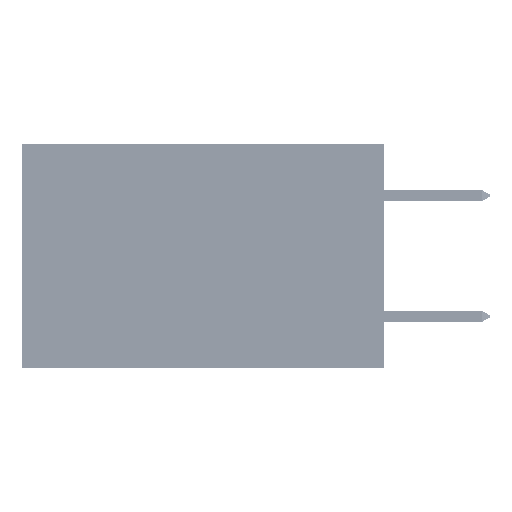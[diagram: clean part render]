
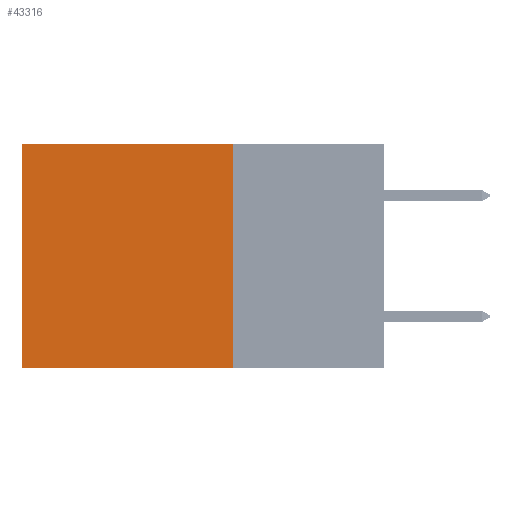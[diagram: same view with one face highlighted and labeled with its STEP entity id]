
A CAD part, left-side view. The second image highlights one B-rep face of the part: STEP entity #43316.
In plain terms, the highlighted planar face has unit normal (-1, 0, 0).
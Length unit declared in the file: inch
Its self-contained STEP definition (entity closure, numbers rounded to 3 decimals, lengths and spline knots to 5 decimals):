
#199 = VERTEX_POINT ( 'NONE', #32326 ) ;
#1847 = PLANE ( 'NONE',  #6595 ) ;
#2545 = VERTEX_POINT ( 'NONE', #3781 ) ;
#2613 = LINE ( 'NONE', #25342, #10153 ) ;
#3607 = ORIENTED_EDGE ( 'NONE', *, *, #38591, .T. ) ;
#3781 = CARTESIAN_POINT ( 'NONE',  ( 0.2875, 0.6, 0. ) ) ;
#4922 = CARTESIAN_POINT ( 'NONE',  ( 0.2875, 0.25, 0. ) ) ;
#6576 = DIRECTION ( 'NONE',  ( 0., 0., -1. ) ) ;
#6595 = AXIS2_PLACEMENT_3D ( 'NONE', #4922, #30850, #41994 ) ;
#10153 = VECTOR ( 'NONE', #14310, 39.37008 ) ;
#14129 = VERTEX_POINT ( 'NONE', #35237 ) ;
#14201 = CARTESIAN_POINT ( 'NONE',  ( 0.2875, 0.25, 0. ) ) ;
#14310 = DIRECTION ( 'NONE',  ( 0., 1., 0. ) ) ;
#16188 = FACE_OUTER_BOUND ( 'NONE', #47750, .T. ) ;
#17707 = EDGE_CURVE ( 'NONE', #199, #14129, #29790, .T. ) ;
#20674 = LINE ( 'NONE', #14201, #45599 ) ;
#21449 = DIRECTION ( 'NONE',  ( 0., 0., -1. ) ) ;
#22335 = CARTESIAN_POINT ( 'NONE',  ( 0.2875, 0.25, 0. ) ) ;
#23956 = VECTOR ( 'NONE', #6576, 39.37008 ) ;
#24790 = ORIENTED_EDGE ( 'NONE', *, *, #17707, .F. ) ;
#25342 = CARTESIAN_POINT ( 'NONE',  ( 0.2875, 0.25, 0. ) ) ;
#27481 = VECTOR ( 'NONE', #33454, 39.37008 ) ;
#29182 = ORIENTED_EDGE ( 'NONE', *, *, #36171, .F. ) ;
#29790 = LINE ( 'NONE', #40847, #27481 ) ;
#30850 = DIRECTION ( 'NONE',  ( 1., 0., 0. ) ) ;
#32063 = CARTESIAN_POINT ( 'NONE',  ( 0.2875, 0.6, 0. ) ) ;
#32326 = CARTESIAN_POINT ( 'NONE',  ( 0.2875, 0.25, -0.37 ) ) ;
#33454 = DIRECTION ( 'NONE',  ( 0., 1., 0. ) ) ;
#35237 = CARTESIAN_POINT ( 'NONE',  ( 0.2875, 0.6, -0.37 ) ) ;
#36171 = EDGE_CURVE ( 'NONE', #40647, #199, #20674, .T. ) ;
#38483 = ORIENTED_EDGE ( 'NONE', *, *, #45754, .T. ) ;
#38591 = EDGE_CURVE ( 'NONE', #2545, #14129, #41300, .T. ) ;
#40647 = VERTEX_POINT ( 'NONE', #22335 ) ;
#40847 = CARTESIAN_POINT ( 'NONE',  ( 0.2875, 0.25, -0.37 ) ) ;
#41300 = LINE ( 'NONE', #32063, #23956 ) ;
#41994 = DIRECTION ( 'NONE',  ( 0., 0., -1. ) ) ;
#43316 = ADVANCED_FACE ( 'NONE', ( #16188 ), #1847, .F. ) ;
#45599 = VECTOR ( 'NONE', #21449, 39.37008 ) ;
#45754 = EDGE_CURVE ( 'NONE', #40647, #2545, #2613, .T. ) ;
#47750 = EDGE_LOOP ( 'NONE', ( #3607, #24790, #29182, #38483 ) ) ;
